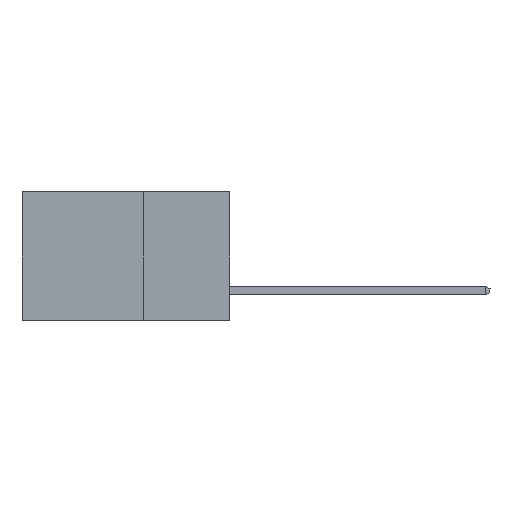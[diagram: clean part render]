
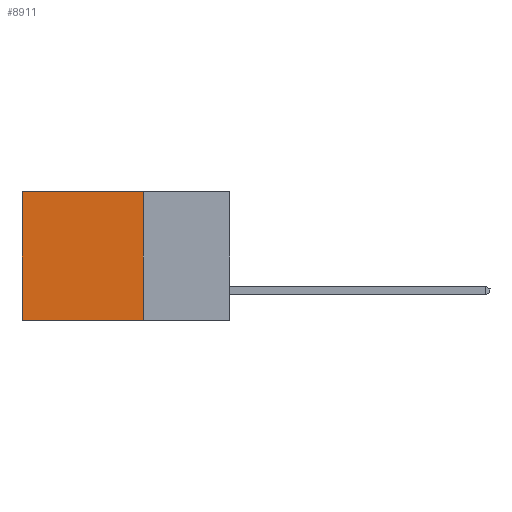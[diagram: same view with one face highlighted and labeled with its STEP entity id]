
A CAD part, left-side view. The second image highlights one B-rep face of the part: STEP entity #8911.
In plain terms, the highlighted planar face has unit normal (-1, 0, 0).
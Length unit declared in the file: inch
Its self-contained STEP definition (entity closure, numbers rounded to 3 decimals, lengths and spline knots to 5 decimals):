
#92 = ORIENTED_EDGE ( 'NONE', *, *, #10608, .F. ) ;
#222 = VERTEX_POINT ( 'NONE', #11892 ) ;
#1855 = ORIENTED_EDGE ( 'NONE', *, *, #6923, .T. ) ;
#1873 = LINE ( 'NONE', #4278, #5758 ) ;
#2266 = DIRECTION ( 'NONE',  ( 0., 0., -1. ) ) ;
#3713 = VERTEX_POINT ( 'NONE', #12890 ) ;
#3729 = FACE_OUTER_BOUND ( 'NONE', #10158, .T. ) ;
#4277 = CARTESIAN_POINT ( 'NONE',  ( 0.2615, 0.25, 0. ) ) ;
#4278 = CARTESIAN_POINT ( 'NONE',  ( 0.2615, 0.25, -0.37 ) ) ;
#4397 = VECTOR ( 'NONE', #8167, 39.37008 ) ;
#4920 = CARTESIAN_POINT ( 'NONE',  ( 0.2615, 0.6, -0.37 ) ) ;
#5758 = VECTOR ( 'NONE', #8151, 39.37008 ) ;
#5999 = CARTESIAN_POINT ( 'NONE',  ( 0.2615, 0.25, -0.37 ) ) ;
#6426 = VECTOR ( 'NONE', #2266, 39.37008 ) ;
#6923 = EDGE_CURVE ( 'NONE', #3713, #12982, #8540, .T. ) ;
#7208 = PLANE ( 'NONE',  #14314 ) ;
#7361 = EDGE_CURVE ( 'NONE', #12112, #3713, #15767, .T. ) ;
#7950 = VECTOR ( 'NONE', #13207, 39.37008 ) ;
#8151 = DIRECTION ( 'NONE',  ( 0., 0., -1. ) ) ;
#8167 = DIRECTION ( 'NONE',  ( 0., 1., 0. ) ) ;
#8540 = LINE ( 'NONE', #4920, #6426 ) ;
#8654 = DIRECTION ( 'NONE',  ( 1., 0., 0. ) ) ;
#8911 = ADVANCED_FACE ( 'NONE', ( #3729 ), #7208, .F. ) ;
#10158 = EDGE_LOOP ( 'NONE', ( #1855, #92, #10974, #10737 ) ) ;
#10535 = LINE ( 'NONE', #14190, #4397 ) ;
#10608 = EDGE_CURVE ( 'NONE', #222, #12982, #10535, .T. ) ;
#10737 = ORIENTED_EDGE ( 'NONE', *, *, #7361, .T. ) ;
#10974 = ORIENTED_EDGE ( 'NONE', *, *, #14782, .F. ) ;
#11892 = CARTESIAN_POINT ( 'NONE',  ( 0.2615, 0.25, -0.37 ) ) ;
#12112 = VERTEX_POINT ( 'NONE', #4277 ) ;
#12250 = CARTESIAN_POINT ( 'NONE',  ( 0.2615, 0.25, 0. ) ) ;
#12890 = CARTESIAN_POINT ( 'NONE',  ( 0.2615, 0.6, 0. ) ) ;
#12982 = VERTEX_POINT ( 'NONE', #13727 ) ;
#13207 = DIRECTION ( 'NONE',  ( 0., 1., 0. ) ) ;
#13727 = CARTESIAN_POINT ( 'NONE',  ( 0.2615, 0.6, -0.37 ) ) ;
#14190 = CARTESIAN_POINT ( 'NONE',  ( 0.2615, 0.25, -0.37 ) ) ;
#14314 = AXIS2_PLACEMENT_3D ( 'NONE', #5999, #8654, #14449 ) ;
#14449 = DIRECTION ( 'NONE',  ( 0., 0., -1. ) ) ;
#14782 = EDGE_CURVE ( 'NONE', #12112, #222, #1873, .T. ) ;
#15767 = LINE ( 'NONE', #12250, #7950 ) ;
